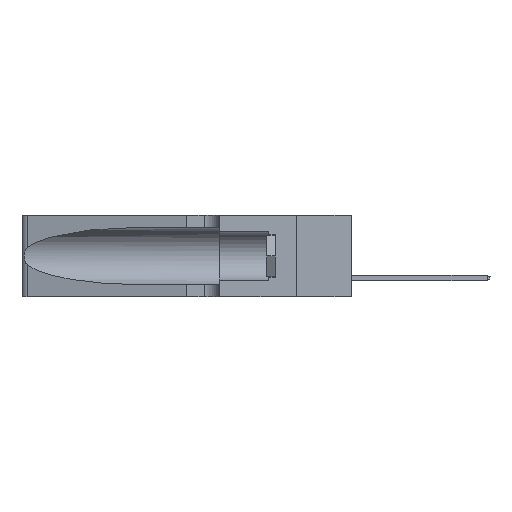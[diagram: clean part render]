
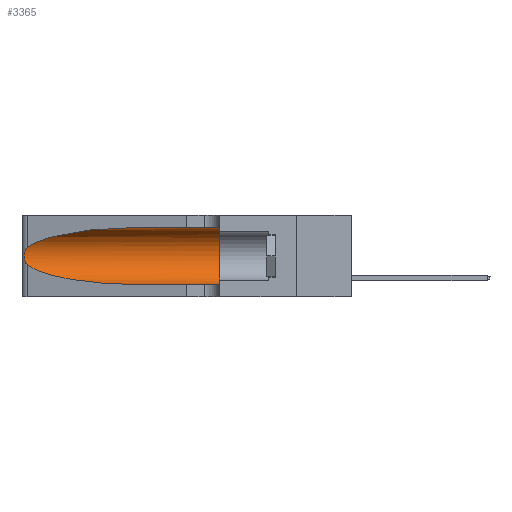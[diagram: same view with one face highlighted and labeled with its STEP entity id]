
A CAD part, left-side view. The second image highlights one B-rep face of the part: STEP entity #3365.
In plain terms, the highlighted cylindrical face has radius 3.308 mm (diameter 6.617 mm), a partial arc.
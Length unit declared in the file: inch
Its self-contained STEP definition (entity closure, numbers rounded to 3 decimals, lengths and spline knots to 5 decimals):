
#82 = ORIENTED_EDGE ( 'NONE', *, *, #47600, .F. ) ;
#539 = CARTESIAN_POINT ( 'NONE',  ( 0.25787, 1.23484, 0.2124 ) ) ;
#700 = CARTESIAN_POINT ( 'NONE',  ( 0.25639, 1.23186, 0.15144 ) ) ;
#915 = CARTESIAN_POINT ( 'NONE',  ( 0.25487, 1.22718, 0.14631 ) ) ;
#2423 = EDGE_CURVE ( 'NONE', #46873, #23521, #44666, .T. ) ;
#2682 = CARTESIAN_POINT ( 'NONE',  ( 0.1305, 0.35, 0.31525 ) ) ;
#2821 = DIRECTION ( 'NONE',  ( 0., -1., 0. ) ) ;
#3365 = ADVANCED_FACE ( 'NONE', ( #28098 ), #32327, .F. ) ;
#3389 = CARTESIAN_POINT ( 'NONE',  ( 0.18966, 0.96281, 0.31525 ) ) ;
#3533 = DIRECTION ( 'NONE',  ( 0., -1., 0. ) ) ;
#4435 = CARTESIAN_POINT ( 'NONE',  ( 0.26075, 1.23896, 0.19203 ) ) ;
#4745 = CARTESIAN_POINT ( 'NONE',  ( 0.25555, 1.22994, 0.2215 ) ) ;
#4865 = CARTESIAN_POINT ( 'NONE',  ( 0.25487, 1.22718, 0.22369 ) ) ;
#5550 = CIRCLE ( 'NONE', #43349, 0.13025 ) ;
#5684 = CARTESIAN_POINT ( 'NONE',  ( 0.18966, 0.96281, 0.05475 ) ) ;
#8099 = EDGE_LOOP ( 'NONE', ( #34064, #12879, #14460, #36900, #16175, #82 ) ) ;
#8209 = EDGE_CURVE ( 'NONE', #38252, #22720, #33256, .T. ) ;
#8418 = CARTESIAN_POINT ( 'NONE',  ( 0.25555, 1.22993, 0.14849 ) ) ;
#9334 = CARTESIAN_POINT ( 'NONE',  ( 0.2373, 1.15595, 0.08982 ) ) ;
#11218 = CARTESIAN_POINT ( 'NONE',  ( 0.2373, 1.15595, 0.28018 ) ) ;
#12128 = CARTESIAN_POINT ( 'NONE',  ( 0.25854, 1.2359, 0.20912 ) ) ;
#12879 = ORIENTED_EDGE ( 'NONE', *, *, #36792, .T. ) ;
#13019 = CARTESIAN_POINT ( 'NONE',  ( 0.1305, 0.35, 0.185 ) ) ;
#13393 = CARTESIAN_POINT ( 'NONE',  ( 0.1305, 0.72297, 0.31525 ) ) ;
#14056 = B_SPLINE_CURVE_WITH_KNOTS ( 'NONE', 3,
 ( #23588, #4745, #27647, #539, #12128, #27497, #4435, #43127, #31365, #42979, #23734, #700, #8418, #35386 ),
 .UNSPECIFIED., .F., .F.,
 ( 4, 2, 2, 2, 2, 2, 4 ),
 ( 0., 0.00027, 0.00053, 0.00107, 0.0016, 0.00187, 0.00214 ),
 .UNSPECIFIED. ) ;
#14460 = ORIENTED_EDGE ( 'NONE', *, *, #2423, .T. ) ;
#16175 = ORIENTED_EDGE ( 'NONE', *, *, #22949, .F. ) ;
#16689 = CARTESIAN_POINT ( 'NONE',  ( 0.1305, 0.72297, 0.05475 ) ) ;
#22324 = CARTESIAN_POINT ( 'NONE',  ( 0.1305, 0.72297, 0.31525 ) ) ;
#22688 = CARTESIAN_POINT ( 'NONE',  ( 0.1305, 1.61858, 0.185 ) ) ;
#22720 = VERTEX_POINT ( 'NONE', #4865 ) ;
#22949 = EDGE_CURVE ( 'NONE', #42206, #25453, #5550, .T. ) ;
#23521 = VERTEX_POINT ( 'NONE', #37067 ) ;
#23588 = CARTESIAN_POINT ( 'NONE',  ( 0.25487, 1.22718, 0.22369 ) ) ;
#23734 = CARTESIAN_POINT ( 'NONE',  ( 0.25789, 1.23486, 0.15765 ) ) ;
#25453 = VERTEX_POINT ( 'NONE', #39617 ) ;
#26420 = CARTESIAN_POINT ( 'NONE',  ( 0.1305, 1.61858, 0.05475 ) ) ;
#26486 = VECTOR ( 'NONE', #2821, 39.37008 ) ;
#26750 = CARTESIAN_POINT ( 'NONE',  ( 0.25487, 1.22718, 0.22369 ) ) ;
#27497 = CARTESIAN_POINT ( 'NONE',  ( 0.26018, 1.23835, 0.19895 ) ) ;
#27647 = CARTESIAN_POINT ( 'NONE',  ( 0.25639, 1.23184, 0.21858 ) ) ;
#28098 = FACE_OUTER_BOUND ( 'NONE', #8099, .T. ) ;
#28764 = DIRECTION ( 'NONE',  ( 0., 1., 0. ) ) ;
#30487 = DIRECTION ( 'NONE',  ( 0., -1., 0. ) ) ;
#30503 = LINE ( 'NONE', #26420, #37105 ) ;
#31365 = CARTESIAN_POINT ( 'NONE',  ( 0.26017, 1.23833, 0.17102 ) ) ;
#31889 = CARTESIAN_POINT ( 'NONE',  ( 0.25487, 1.22718, 0.14631 ) ) ;
#32327 = CYLINDRICAL_SURFACE ( 'NONE', #46197, 0.13025 ) ;
#33256 =( BOUNDED_CURVE ( )  B_SPLINE_CURVE ( 3, ( #22324, #3389, #11218, #26750 ),
 .UNSPECIFIED., .F., .F. ) 
 B_SPLINE_CURVE_WITH_KNOTS ( ( 4, 4 ),
 ( 1.5708, 2.84003 ),
 .UNSPECIFIED. ) 
 CURVE ( )  GEOMETRIC_REPRESENTATION_ITEM ( )  RATIONAL_B_SPLINE_CURVE ( ( 1., 0.87, 0.87, 1. ) ) 
 REPRESENTATION_ITEM ( '' )  );
#34064 = ORIENTED_EDGE ( 'NONE', *, *, #8209, .T. ) ;
#35386 = CARTESIAN_POINT ( 'NONE',  ( 0.25487, 1.22718, 0.14631 ) ) ;
#36672 = LINE ( 'NONE', #44882, #26486 ) ;
#36792 = EDGE_CURVE ( 'NONE', #22720, #46873, #14056, .T. ) ;
#36900 = ORIENTED_EDGE ( 'NONE', *, *, #49699, .T. ) ;
#37067 = CARTESIAN_POINT ( 'NONE',  ( 0.1305, 0.72297, 0.05475 ) ) ;
#37105 = VECTOR ( 'NONE', #3533, 39.37008 ) ;
#38252 = VERTEX_POINT ( 'NONE', #13393 ) ;
#39617 = CARTESIAN_POINT ( 'NONE',  ( 0.1305, 0.35, 0.05475 ) ) ;
#40603 = DIRECTION ( 'NONE',  ( 0., 0., 1. ) ) ;
#42090 = DIRECTION ( 'NONE',  ( 0., 0., -1. ) ) ;
#42206 = VERTEX_POINT ( 'NONE', #2682 ) ;
#42979 = CARTESIAN_POINT ( 'NONE',  ( 0.25856, 1.23593, 0.16098 ) ) ;
#43127 = CARTESIAN_POINT ( 'NONE',  ( 0.26075, 1.23896, 0.178 ) ) ;
#43349 = AXIS2_PLACEMENT_3D ( 'NONE', #13019, #28764, #40603 ) ;
#44666 =( BOUNDED_CURVE ( )  B_SPLINE_CURVE ( 3, ( #915, #9334, #5684, #16689 ),
 .UNSPECIFIED., .F., .F. ) 
 B_SPLINE_CURVE_WITH_KNOTS ( ( 4, 4 ),
 ( 3.44316, 4.71239 ),
 .UNSPECIFIED. ) 
 CURVE ( )  GEOMETRIC_REPRESENTATION_ITEM ( )  RATIONAL_B_SPLINE_CURVE ( ( 1., 0.87, 0.87, 1. ) ) 
 REPRESENTATION_ITEM ( '' )  );
#44882 = CARTESIAN_POINT ( 'NONE',  ( 0.1305, 1.61858, 0.31525 ) ) ;
#46197 = AXIS2_PLACEMENT_3D ( 'NONE', #22688, #30487, #42090 ) ;
#46873 = VERTEX_POINT ( 'NONE', #31889 ) ;
#47600 = EDGE_CURVE ( 'NONE', #38252, #42206, #36672, .T. ) ;
#49699 = EDGE_CURVE ( 'NONE', #23521, #25453, #30503, .T. ) ;
